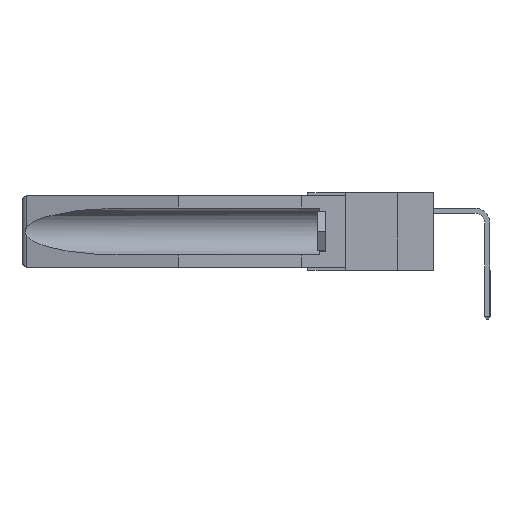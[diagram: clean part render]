
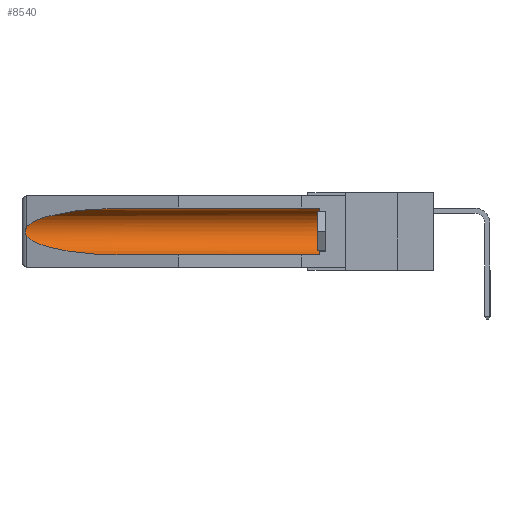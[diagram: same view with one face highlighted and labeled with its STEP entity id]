
A CAD part, left-side view. The second image highlights one B-rep face of the part: STEP entity #8540.
In plain terms, the highlighted cylindrical face has radius 2.857 mm (diameter 5.715 mm), a partial arc.
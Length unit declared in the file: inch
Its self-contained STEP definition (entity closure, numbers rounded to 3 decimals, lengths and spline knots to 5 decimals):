
#25 = CARTESIAN_POINT ( 'NONE',  ( 0.26597, 1.52961, -0.15275 ) ) ;
#632 = CARTESIAN_POINT ( 'NONE',  ( 0.155, 0.126, -0.1715 ) ) ;
#998 = CARTESIAN_POINT ( 'NONE',  ( 0.155, 0.126, -0.059 ) ) ;
#1527 = CARTESIAN_POINT ( 'NONE',  ( 0.26537, 1.52718, -0.14972 ) ) ;
#1580 = VERTEX_POINT ( 'NONE', #998 ) ;
#1764 = CARTESIAN_POINT ( 'NONE',  ( 0.25451, 1.48313, -0.09465 ) ) ;
#1822 = VERTEX_POINT ( 'NONE', #4261 ) ;
#1870 = CARTESIAN_POINT ( 'NONE',  ( 0.2673, 1.53269, -0.17917 ) ) ;
#2102 = EDGE_CURVE ( 'NONE', #16239, #10224, #12277, .T. ) ;
#2401 = EDGE_CURVE ( 'NONE', #1822, #1580, #16879, .T. ) ;
#3204 = CARTESIAN_POINT ( 'NONE',  ( 0.155, 1.07973, -0.059 ) ) ;
#3220 = EDGE_CURVE ( 'NONE', #6937, #14979, #18141, .T. ) ;
#3842 = VECTOR ( 'NONE', #11968, 39.37008 ) ;
#4174 = CARTESIAN_POINT ( 'NONE',  ( 0.2675, 1.53308, -0.16763 ) ) ;
#4261 = CARTESIAN_POINT ( 'NONE',  ( 0.155, 0.126, -0.284 ) ) ;
#4485 = CARTESIAN_POINT ( 'NONE',  ( 0.2675, 1.53308, -0.17534 ) ) ;
#4901 = CARTESIAN_POINT ( 'NONE',  ( 0.155, -0.30754, -0.284 ) ) ;
#5033 = DIRECTION ( 'NONE',  ( 0., 0., 1. ) ) ;
#5900 = EDGE_CURVE ( 'NONE', #1580, #6937, #17981, .T. ) ;
#6937 = VERTEX_POINT ( 'NONE', #3204 ) ;
#7088 = ORIENTED_EDGE ( 'NONE', *, *, #2102, .T. ) ;
#7225 = AXIS2_PLACEMENT_3D ( 'NONE', #12180, #16510, #7909 ) ;
#7654 = CARTESIAN_POINT ( 'NONE',  ( 0.26655, 1.53094, -0.18657 ) ) ;
#7909 = DIRECTION ( 'NONE',  ( 0., 0., 1. ) ) ;
#7986 = CARTESIAN_POINT ( 'NONE',  ( 0.25451, 1.48313, -0.24835 ) ) ;
#8085 = EDGE_CURVE ( 'NONE', #1822, #10224, #17466, .T. ) ;
#8540 = ADVANCED_FACE ( 'NONE', ( #15417 ), #14315, .F. ) ;
#8761 = B_SPLINE_CURVE_WITH_KNOTS ( 'NONE', 3,
 ( #12957, #25, #10014, #12783, #4174, #4485, #1870, #7654, #11800, #9047 ),
 .UNSPECIFIED., .F., .F.,
 ( 4, 2, 2, 2, 4 ),
 ( 0., 0.00029, 0.00058, 0.00087, 0.00117 ),
 .UNSPECIFIED. ) ;
#8990 = CARTESIAN_POINT ( 'NONE',  ( 0.155, 1.07973, -0.059 ) ) ;
#9047 = CARTESIAN_POINT ( 'NONE',  ( 0.26537, 1.52718, -0.19328 ) ) ;
#9284 = DIRECTION ( 'NONE',  ( 0., 1., 0. ) ) ;
#9428 = DIRECTION ( 'NONE',  ( 0., -1., 0. ) ) ;
#9453 = CARTESIAN_POINT ( 'NONE',  ( 0.21114, 1.30732, -0.284 ) ) ;
#9467 = EDGE_LOOP ( 'NONE', ( #12297, #9853, #7088, #15503, #16129, #16557 ) ) ;
#9853 = ORIENTED_EDGE ( 'NONE', *, *, #17536, .T. ) ;
#10014 = CARTESIAN_POINT ( 'NONE',  ( 0.26654, 1.53092, -0.15636 ) ) ;
#10224 = VERTEX_POINT ( 'NONE', #11094 ) ;
#10867 = CARTESIAN_POINT ( 'NONE',  ( 0.155, 1.07973, -0.284 ) ) ;
#11094 = CARTESIAN_POINT ( 'NONE',  ( 0.155, 1.07973, -0.284 ) ) ;
#11495 = AXIS2_PLACEMENT_3D ( 'NONE', #632, #9428, #5033 ) ;
#11800 = CARTESIAN_POINT ( 'NONE',  ( 0.26597, 1.5296, -0.19026 ) ) ;
#11968 = DIRECTION ( 'NONE',  ( 0., 1., 0. ) ) ;
#12180 = CARTESIAN_POINT ( 'NONE',  ( 0.155, -0.30754, -0.1715 ) ) ;
#12277 =( BOUNDED_CURVE ( )  B_SPLINE_CURVE ( 3, ( #13793, #7986, #9453, #10867 ),
 .UNSPECIFIED., .F., .F. ) 
 B_SPLINE_CURVE_WITH_KNOTS ( ( 4, 4 ),
 ( 0.1948, 1.5708 ),
 .UNSPECIFIED. ) 
 CURVE ( )  GEOMETRIC_REPRESENTATION_ITEM ( )  RATIONAL_B_SPLINE_CURVE ( ( 1., 0.848, 0.848, 1. ) ) 
 REPRESENTATION_ITEM ( '' )  );
#12297 = ORIENTED_EDGE ( 'NONE', *, *, #3220, .T. ) ;
#12783 = CARTESIAN_POINT ( 'NONE',  ( 0.2673, 1.5327, -0.16383 ) ) ;
#12957 = CARTESIAN_POINT ( 'NONE',  ( 0.26537, 1.52718, -0.14972 ) ) ;
#13793 = CARTESIAN_POINT ( 'NONE',  ( 0.26537, 1.52718, -0.19328 ) ) ;
#14315 = CYLINDRICAL_SURFACE ( 'NONE', #7225, 0.1125 ) ;
#14376 = CARTESIAN_POINT ( 'NONE',  ( 0.26537, 1.52718, -0.19328 ) ) ;
#14763 = CARTESIAN_POINT ( 'NONE',  ( 0.21114, 1.30732, -0.059 ) ) ;
#14979 = VERTEX_POINT ( 'NONE', #1527 ) ;
#15417 = FACE_OUTER_BOUND ( 'NONE', #9467, .T. ) ;
#15503 = ORIENTED_EDGE ( 'NONE', *, *, #8085, .F. ) ;
#15651 = VECTOR ( 'NONE', #9284, 39.37008 ) ;
#16129 = ORIENTED_EDGE ( 'NONE', *, *, #2401, .T. ) ;
#16200 = CARTESIAN_POINT ( 'NONE',  ( 0.26537, 1.52718, -0.14972 ) ) ;
#16239 = VERTEX_POINT ( 'NONE', #14376 ) ;
#16510 = DIRECTION ( 'NONE',  ( 0., 1., 0. ) ) ;
#16557 = ORIENTED_EDGE ( 'NONE', *, *, #5900, .T. ) ;
#16879 = CIRCLE ( 'NONE', #11495, 0.1125 ) ;
#17466 = LINE ( 'NONE', #4901, #15651 ) ;
#17536 = EDGE_CURVE ( 'NONE', #14979, #16239, #8761, .T. ) ;
#17827 = CARTESIAN_POINT ( 'NONE',  ( 0.155, -0.30754, -0.059 ) ) ;
#17981 = LINE ( 'NONE', #17827, #3842 ) ;
#18141 =( BOUNDED_CURVE ( )  B_SPLINE_CURVE ( 3, ( #8990, #14763, #1764, #16200 ),
 .UNSPECIFIED., .F., .T. ) 
 B_SPLINE_CURVE_WITH_KNOTS ( ( 4, 4 ),
 ( 4.71239, 6.08839 ),
 .UNSPECIFIED. ) 
 CURVE ( )  GEOMETRIC_REPRESENTATION_ITEM ( )  RATIONAL_B_SPLINE_CURVE ( ( 1., 0.848, 0.848, 1. ) ) 
 REPRESENTATION_ITEM ( '' )  );
